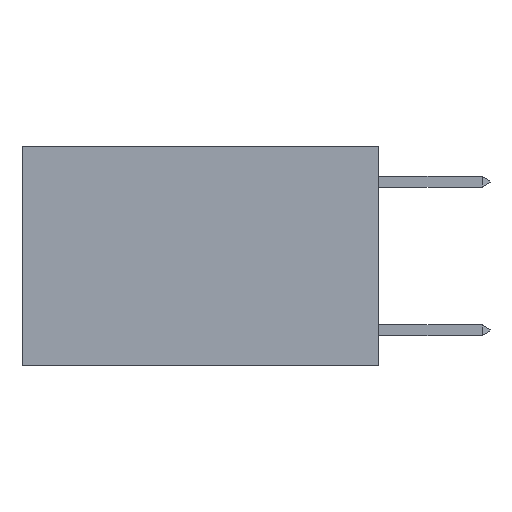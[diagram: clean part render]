
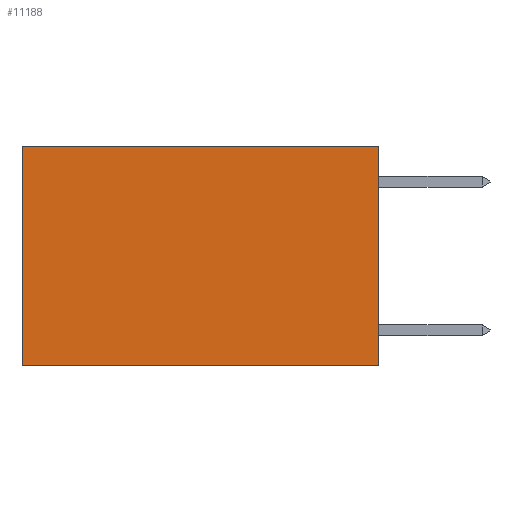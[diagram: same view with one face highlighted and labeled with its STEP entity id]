
A CAD part, left-side view. The second image highlights one B-rep face of the part: STEP entity #11188.
In plain terms, the highlighted planar face has unit normal (-1, 0, 0).
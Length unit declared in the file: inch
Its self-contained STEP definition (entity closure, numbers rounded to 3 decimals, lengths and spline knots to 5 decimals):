
#67 = DIRECTION ( 'NONE',  ( 0., 0., -1. ) ) ;
#294 = CARTESIAN_POINT ( 'NONE',  ( 0.2625, 0., -0.37 ) ) ;
#849 = LINE ( 'NONE', #7673, #7289 ) ;
#1073 = DIRECTION ( 'NONE',  ( 0., 1., 0. ) ) ;
#1280 = VERTEX_POINT ( 'NONE', #5838 ) ;
#1285 = CARTESIAN_POINT ( 'NONE',  ( 0.2625, 0., 0. ) ) ;
#1692 = EDGE_CURVE ( 'NONE', #6783, #3052, #10484, .T. ) ;
#1828 = VERTEX_POINT ( 'NONE', #294 ) ;
#2197 = EDGE_CURVE ( 'NONE', #1828, #3052, #849, .T. ) ;
#2236 = FACE_OUTER_BOUND ( 'NONE', #8766, .T. ) ;
#3052 = VERTEX_POINT ( 'NONE', #9636 ) ;
#3119 = ORIENTED_EDGE ( 'NONE', *, *, #6924, .F. ) ;
#4262 = DIRECTION ( 'NONE',  ( 1., 0., 0. ) ) ;
#4432 = CARTESIAN_POINT ( 'NONE',  ( 0.2625, 0.6, 0. ) ) ;
#4877 = CARTESIAN_POINT ( 'NONE',  ( 0.2625, 0.6, 0. ) ) ;
#4941 = PLANE ( 'NONE',  #8570 ) ;
#5251 = CARTESIAN_POINT ( 'NONE',  ( 0.2625, 0., 0. ) ) ;
#5838 = CARTESIAN_POINT ( 'NONE',  ( 0.2625, 0., 0. ) ) ;
#5848 = LINE ( 'NONE', #11384, #10121 ) ;
#6783 = VERTEX_POINT ( 'NONE', #4432 ) ;
#6924 = EDGE_CURVE ( 'NONE', #1280, #1828, #10912, .T. ) ;
#7289 = VECTOR ( 'NONE', #9427, 39.37008 ) ;
#7439 = ORIENTED_EDGE ( 'NONE', *, *, #1692, .T. ) ;
#7673 = CARTESIAN_POINT ( 'NONE',  ( 0.2625, 0., -0.37 ) ) ;
#8034 = VECTOR ( 'NONE', #67, 39.37008 ) ;
#8570 = AXIS2_PLACEMENT_3D ( 'NONE', #1285, #4262, #11541 ) ;
#8766 = EDGE_LOOP ( 'NONE', ( #7439, #10014, #3119, #12097 ) ) ;
#8987 = DIRECTION ( 'NONE',  ( 0., 0., -1. ) ) ;
#8992 = EDGE_CURVE ( 'NONE', #1280, #6783, #5848, .T. ) ;
#9427 = DIRECTION ( 'NONE',  ( 0., 1., 0. ) ) ;
#9636 = CARTESIAN_POINT ( 'NONE',  ( 0.2625, 0.6, -0.37 ) ) ;
#10014 = ORIENTED_EDGE ( 'NONE', *, *, #2197, .F. ) ;
#10121 = VECTOR ( 'NONE', #1073, 39.37008 ) ;
#10277 = VECTOR ( 'NONE', #8987, 39.37008 ) ;
#10484 = LINE ( 'NONE', #4877, #8034 ) ;
#10912 = LINE ( 'NONE', #5251, #10277 ) ;
#11188 = ADVANCED_FACE ( 'NONE', ( #2236 ), #4941, .F. ) ;
#11384 = CARTESIAN_POINT ( 'NONE',  ( 0.2625, 0., 0. ) ) ;
#11541 = DIRECTION ( 'NONE',  ( 0., 0., -1. ) ) ;
#12097 = ORIENTED_EDGE ( 'NONE', *, *, #8992, .T. ) ;
